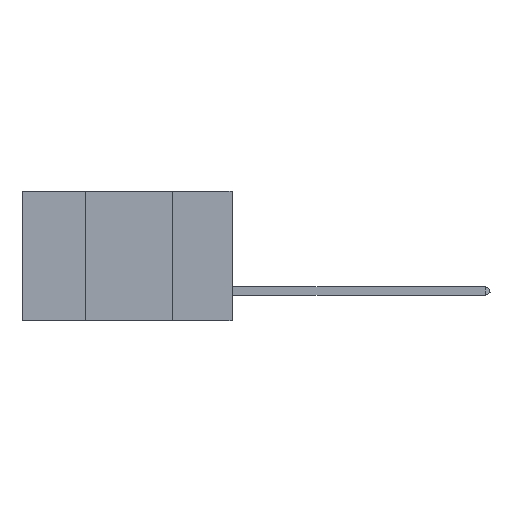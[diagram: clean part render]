
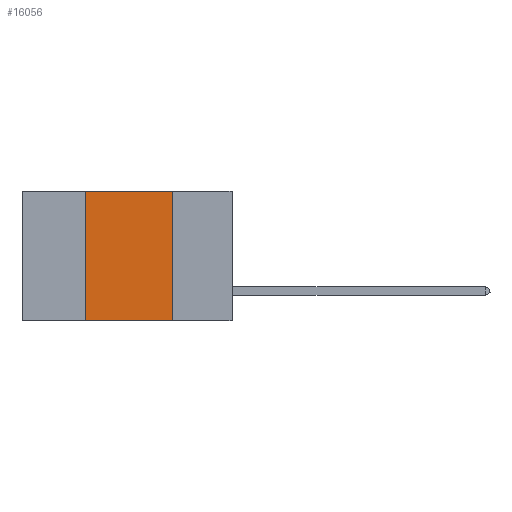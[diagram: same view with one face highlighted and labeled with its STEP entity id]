
A CAD part, left-side view. The second image highlights one B-rep face of the part: STEP entity #16056.
In plain terms, the highlighted planar face has unit normal (-1, 0, 0).
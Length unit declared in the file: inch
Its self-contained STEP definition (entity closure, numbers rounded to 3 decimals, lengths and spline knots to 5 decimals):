
#281 = ORIENTED_EDGE ( 'NONE', *, *, #19266, .F. ) ;
#403 = CARTESIAN_POINT ( 'NONE',  ( 0., 0.17, 0. ) ) ;
#1708 = VERTEX_POINT ( 'NONE', #15676 ) ;
#2417 = CARTESIAN_POINT ( 'NONE',  ( 0., 0.42, 0. ) ) ;
#3090 = ORIENTED_EDGE ( 'NONE', *, *, #21338, .F. ) ;
#3361 = DIRECTION ( 'NONE',  ( 0., 0., 1. ) ) ;
#4155 = LINE ( 'NONE', #21981, #9863 ) ;
#4159 = LINE ( 'NONE', #10532, #20945 ) ;
#4223 = CARTESIAN_POINT ( 'NONE',  ( 0., 0.6, 0. ) ) ;
#4745 = DIRECTION ( 'NONE',  ( 1., 0., 0. ) ) ;
#5275 = ORIENTED_EDGE ( 'NONE', *, *, #20324, .T. ) ;
#5961 = DIRECTION ( 'NONE',  ( 0., -1., 0. ) ) ;
#6229 = LINE ( 'NONE', #14472, #11376 ) ;
#6537 = VECTOR ( 'NONE', #5961, 39.37008 ) ;
#7395 = AXIS2_PLACEMENT_3D ( 'NONE', #9605, #4745, #20057 ) ;
#7507 = DIRECTION ( 'NONE',  ( 0., 0., -1. ) ) ;
#7847 = VERTEX_POINT ( 'NONE', #403 ) ;
#8013 = PLANE ( 'NONE',  #7395 ) ;
#8094 = DIRECTION ( 'NONE',  ( 0., -1., 0. ) ) ;
#9605 = CARTESIAN_POINT ( 'NONE',  ( 0., 0.6, 0. ) ) ;
#9863 = VECTOR ( 'NONE', #8094, 39.37008 ) ;
#10532 = CARTESIAN_POINT ( 'NONE',  ( 0., 0.42, 0. ) ) ;
#11376 = VECTOR ( 'NONE', #7507, 39.37008 ) ;
#12326 = EDGE_CURVE ( 'NONE', #18060, #7847, #12769, .T. ) ;
#12769 = LINE ( 'NONE', #4223, #6537 ) ;
#14472 = CARTESIAN_POINT ( 'NONE',  ( 0., 0.17, 0. ) ) ;
#14709 = EDGE_LOOP ( 'NONE', ( #3090, #16801, #281, #5275 ) ) ;
#14891 = FACE_OUTER_BOUND ( 'NONE', #14709, .T. ) ;
#15083 = VERTEX_POINT ( 'NONE', #17288 ) ;
#15676 = CARTESIAN_POINT ( 'NONE',  ( 0., 0.17, -0.37 ) ) ;
#16056 = ADVANCED_FACE ( 'NONE', ( #14891 ), #8013, .F. ) ;
#16801 = ORIENTED_EDGE ( 'NONE', *, *, #12326, .F. ) ;
#17288 = CARTESIAN_POINT ( 'NONE',  ( 0., 0.42, -0.37 ) ) ;
#18060 = VERTEX_POINT ( 'NONE', #2417 ) ;
#19266 = EDGE_CURVE ( 'NONE', #15083, #18060, #4159, .T. ) ;
#20057 = DIRECTION ( 'NONE',  ( 0., 0., -1. ) ) ;
#20324 = EDGE_CURVE ( 'NONE', #15083, #1708, #4155, .T. ) ;
#20945 = VECTOR ( 'NONE', #3361, 39.37008 ) ;
#21338 = EDGE_CURVE ( 'NONE', #7847, #1708, #6229, .T. ) ;
#21981 = CARTESIAN_POINT ( 'NONE',  ( 0., 0.6, -0.37 ) ) ;
